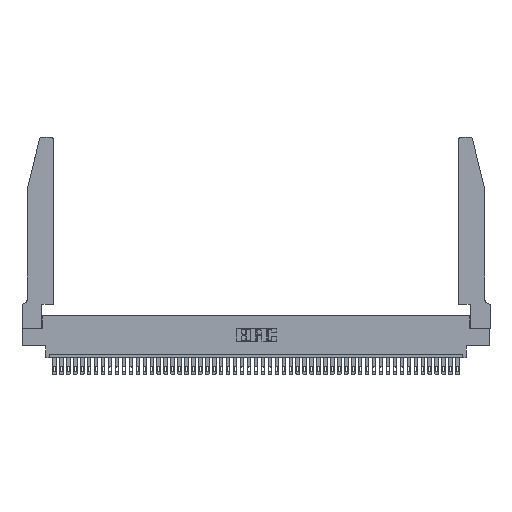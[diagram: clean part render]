
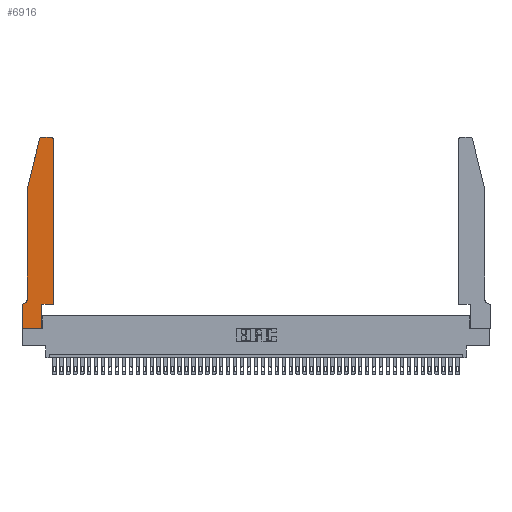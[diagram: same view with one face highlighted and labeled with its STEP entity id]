
A CAD part, top view. The second image highlights one B-rep face of the part: STEP entity #6916.
In plain terms, the highlighted planar face has unit normal (0, 0, 1).
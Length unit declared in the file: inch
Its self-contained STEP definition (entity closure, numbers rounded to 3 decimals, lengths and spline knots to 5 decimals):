
#1205 = CARTESIAN_POINT ( 'NONE',  ( 0.2865, 0.35, 0.37 ) ) ;
#1339 = DIRECTION ( 'NONE',  ( -1., 0., 0. ) ) ;
#1355 = VERTEX_POINT ( 'NONE', #2195 ) ;
#1371 = LINE ( 'NONE', #23516, #34213 ) ;
#1387 = CARTESIAN_POINT ( 'NONE',  ( 0.2865, 0., 0.37 ) ) ;
#1515 = CARTESIAN_POINT ( 'NONE',  ( 0.0755, 0.35, 0.37 ) ) ;
#1694 = VERTEX_POINT ( 'NONE', #45749 ) ;
#1882 = DIRECTION ( 'NONE',  ( 0., -1., 0. ) ) ;
#2130 = VECTOR ( 'NONE', #44470, 39.37008 ) ;
#2163 = DIRECTION ( 'NONE',  ( 0., 0., 1. ) ) ;
#2195 = CARTESIAN_POINT ( 'NONE',  ( 0.4505, 0.35, 0.37 ) ) ;
#2196 = DIRECTION ( 'NONE',  ( 1., 0., 0. ) ) ;
#2375 = EDGE_CURVE ( 'NONE', #15083, #1694, #1371, .T. ) ;
#3679 = CARTESIAN_POINT ( 'NONE',  ( 0.284, 2.75, 0.37 ) ) ;
#3885 = ORIENTED_EDGE ( 'NONE', *, *, #14057, .T. ) ;
#3898 = ORIENTED_EDGE ( 'NONE', *, *, #44945, .T. ) ;
#3936 = DIRECTION ( 'NONE',  ( 0., 1., 0. ) ) ;
#4836 = DIRECTION ( 'NONE',  ( 0., 1., 0. ) ) ;
#5791 = DIRECTION ( 'NONE',  ( 1., 0., 0. ) ) ;
#6006 = EDGE_CURVE ( 'NONE', #31617, #17422, #32103, .T. ) ;
#6017 = EDGE_CURVE ( 'NONE', #23430, #15083, #24167, .T. ) ;
#6916 = ADVANCED_FACE ( 'NONE', ( #33671 ), #13114, .T. ) ;
#9992 = VECTOR ( 'NONE', #30496, 39.37008 ) ;
#11536 = CARTESIAN_POINT ( 'NONE',  ( 0.4505, 0.35, 0.37 ) ) ;
#11774 = DIRECTION ( 'NONE',  ( 0., 0., -1. ) ) ;
#12005 = VERTEX_POINT ( 'NONE', #31058 ) ;
#12359 = CIRCLE ( 'NONE', #36033, 0.03 ) ;
#12542 = LINE ( 'NONE', #33314, #33509 ) ;
#12885 = LINE ( 'NONE', #11536, #2130 ) ;
#13114 = PLANE ( 'NONE',  #22602 ) ;
#13949 = ORIENTED_EDGE ( 'NONE', *, *, #35903, .T. ) ;
#14057 = EDGE_CURVE ( 'NONE', #12005, #44389, #12542, .T. ) ;
#14509 = EDGE_CURVE ( 'NONE', #29203, #38599, #29505, .T. ) ;
#15083 = VERTEX_POINT ( 'NONE', #22842 ) ;
#15716 = CARTESIAN_POINT ( 'NONE',  ( 0.4505, 2.72, 0.37 ) ) ;
#16685 = DIRECTION ( 'NONE',  ( 0., -1., 0. ) ) ;
#17422 = VERTEX_POINT ( 'NONE', #40196 ) ;
#17548 = EDGE_CURVE ( 'NONE', #38599, #35350, #35431, .T. ) ;
#18148 = AXIS2_PLACEMENT_3D ( 'NONE', #22841, #11774, #1339 ) ;
#18666 = VECTOR ( 'NONE', #3936, 39.37008 ) ;
#18931 = CARTESIAN_POINT ( 'NONE',  ( 0.0755, 2., 0.37 ) ) ;
#20671 = DIRECTION ( 'NONE',  ( 0., 0., 1. ) ) ;
#20880 = EDGE_CURVE ( 'NONE', #30439, #12005, #12359, .T. ) ;
#21229 = EDGE_CURVE ( 'NONE', #1694, #31617, #29913, .T. ) ;
#21475 = ORIENTED_EDGE ( 'NONE', *, *, #6017, .T. ) ;
#22423 = VECTOR ( 'NONE', #4836, 39.37008 ) ;
#22602 = AXIS2_PLACEMENT_3D ( 'NONE', #24026, #20671, #2196 ) ;
#22841 = CARTESIAN_POINT ( 'NONE',  ( 0.0055, 0.42, 0.37 ) ) ;
#22842 = CARTESIAN_POINT ( 'NONE',  ( 0., 0.35, 0.37 ) ) ;
#22846 = EDGE_LOOP ( 'NONE', ( #3885, #42066, #42488, #27962, #13949, #21475, #31842, #39726, #44913, #3898, #34671, #46216 ) ) ;
#23213 = CARTESIAN_POINT ( 'NONE',  ( 0.0755, 0.42, 0.37 ) ) ;
#23430 = VERTEX_POINT ( 'NONE', #32123 ) ;
#23516 = CARTESIAN_POINT ( 'NONE',  ( 0., 0., 0.37 ) ) ;
#24026 = CARTESIAN_POINT ( 'NONE',  ( 0., 0.35, 0.37 ) ) ;
#24167 = LINE ( 'NONE', #1515, #9992 ) ;
#25653 = CARTESIAN_POINT ( 'NONE',  ( 0.4505, 0.35, 0.37 ) ) ;
#25716 = DIRECTION ( 'NONE',  ( -1., 0., 0. ) ) ;
#25726 = CIRCLE ( 'NONE', #18148, 0.07 ) ;
#27327 = CARTESIAN_POINT ( 'NONE',  ( 0.4205, 2.72, 0.37 ) ) ;
#27962 = ORIENTED_EDGE ( 'NONE', *, *, #17548, .T. ) ;
#29203 = VERTEX_POINT ( 'NONE', #32963 ) ;
#29505 = LINE ( 'NONE', #18931, #39691 ) ;
#29524 = DIRECTION ( 'NONE',  ( 1., 0., 0. ) ) ;
#29913 = LINE ( 'NONE', #39995, #38394 ) ;
#30439 = VERTEX_POINT ( 'NONE', #15716 ) ;
#30496 = DIRECTION ( 'NONE',  ( -1., 0., 0. ) ) ;
#30892 = VECTOR ( 'NONE', #1882, 39.37008 ) ;
#31058 = CARTESIAN_POINT ( 'NONE',  ( 0.4205, 2.75, 0.37 ) ) ;
#31617 = VERTEX_POINT ( 'NONE', #1387 ) ;
#31692 = DIRECTION ( 'NONE',  ( 1., 0., 0. ) ) ;
#31842 = ORIENTED_EDGE ( 'NONE', *, *, #2375, .T. ) ;
#32103 = LINE ( 'NONE', #1205, #22423 ) ;
#32123 = CARTESIAN_POINT ( 'NONE',  ( 0.0055, 0.35, 0.37 ) ) ;
#32963 = CARTESIAN_POINT ( 'NONE',  ( 0.25487, 2.72718, 0.37 ) ) ;
#33314 = CARTESIAN_POINT ( 'NONE',  ( 0.2605, 2.75, 0.37 ) ) ;
#33509 = VECTOR ( 'NONE', #25716, 39.37008 ) ;
#33671 = FACE_OUTER_BOUND ( 'NONE', #22846, .T. ) ;
#34213 = VECTOR ( 'NONE', #16685, 39.37008 ) ;
#34671 = ORIENTED_EDGE ( 'NONE', *, *, #41146, .T. ) ;
#34757 = AXIS2_PLACEMENT_3D ( 'NONE', #46089, #35317, #31692 ) ;
#35317 = DIRECTION ( 'NONE',  ( 0., 0., 1. ) ) ;
#35350 = VERTEX_POINT ( 'NONE', #23213 ) ;
#35431 = LINE ( 'NONE', #37642, #30892 ) ;
#35717 = LINE ( 'NONE', #25653, #18666 ) ;
#35903 = EDGE_CURVE ( 'NONE', #35350, #23430, #25726, .T. ) ;
#36033 = AXIS2_PLACEMENT_3D ( 'NONE', #27327, #2163, #5791 ) ;
#36065 = CIRCLE ( 'NONE', #34757, 0.03 ) ;
#37630 = DIRECTION ( 'NONE',  ( -0.239, -0.971, 0. ) ) ;
#37642 = CARTESIAN_POINT ( 'NONE',  ( 0.0755, 2., 0.37 ) ) ;
#38394 = VECTOR ( 'NONE', #29524, 39.37008 ) ;
#38599 = VERTEX_POINT ( 'NONE', #43371 ) ;
#39691 = VECTOR ( 'NONE', #37630, 39.37008 ) ;
#39726 = ORIENTED_EDGE ( 'NONE', *, *, #21229, .T. ) ;
#39995 = CARTESIAN_POINT ( 'NONE',  ( 0., 0., 0.37 ) ) ;
#40196 = CARTESIAN_POINT ( 'NONE',  ( 0.2865, 0.35, 0.37 ) ) ;
#41146 = EDGE_CURVE ( 'NONE', #1355, #30439, #35717, .T. ) ;
#42066 = ORIENTED_EDGE ( 'NONE', *, *, #42825, .T. ) ;
#42488 = ORIENTED_EDGE ( 'NONE', *, *, #14509, .T. ) ;
#42825 = EDGE_CURVE ( 'NONE', #44389, #29203, #36065, .T. ) ;
#43371 = CARTESIAN_POINT ( 'NONE',  ( 0.0755, 2., 0.37 ) ) ;
#44389 = VERTEX_POINT ( 'NONE', #3679 ) ;
#44470 = DIRECTION ( 'NONE',  ( 1., 0., 0. ) ) ;
#44913 = ORIENTED_EDGE ( 'NONE', *, *, #6006, .T. ) ;
#44945 = EDGE_CURVE ( 'NONE', #17422, #1355, #12885, .T. ) ;
#45749 = CARTESIAN_POINT ( 'NONE',  ( 0., 0., 0.37 ) ) ;
#46089 = CARTESIAN_POINT ( 'NONE',  ( 0.284, 2.72, 0.37 ) ) ;
#46216 = ORIENTED_EDGE ( 'NONE', *, *, #20880, .T. ) ;
